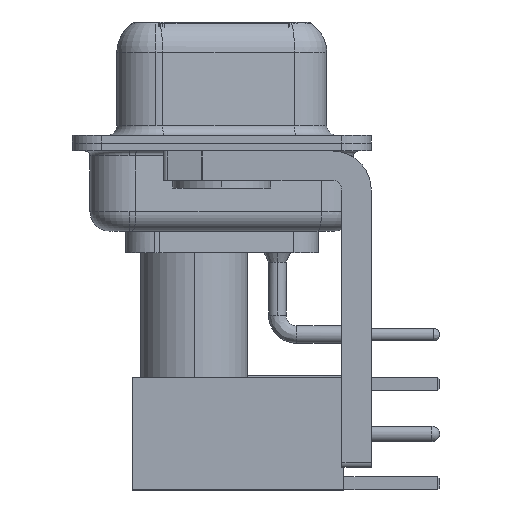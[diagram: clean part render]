
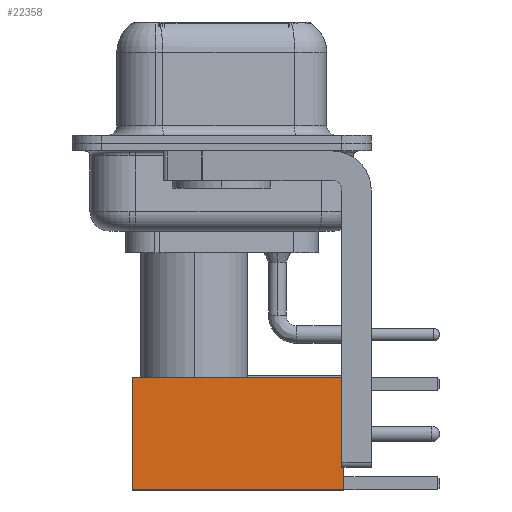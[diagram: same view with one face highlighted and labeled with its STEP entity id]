
A CAD part, left-side view. The second image highlights one B-rep face of the part: STEP entity #22358.
In plain terms, the highlighted face is planar.
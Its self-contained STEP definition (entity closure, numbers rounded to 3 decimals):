
#1876 = LINE ( 'NONE', #10668, #19207 ) ;
#3107 = CARTESIAN_POINT ( 'NONE',  ( 0., 2.875, 0. ) ) ;
#3415 = ORIENTED_EDGE ( 'NONE', *, *, #3549, .F. ) ;
#3437 = VERTEX_POINT ( 'NONE', #18532 ) ;
#3549 = EDGE_CURVE ( 'NONE', #3437, #8320, #31125, .T. ) ;
#3899 = DIRECTION ( 'NONE',  ( 0., 1., 0. ) ) ;
#5084 = EDGE_CURVE ( 'NONE', #8320, #7534, #14195, .T. ) ;
#5472 = DIRECTION ( 'NONE',  ( -1., 0., 0. ) ) ;
#5492 = DIRECTION ( 'NONE',  ( 0., 0., -1. ) ) ;
#7534 = VERTEX_POINT ( 'NONE', #22876 ) ;
#7855 = CARTESIAN_POINT ( 'NONE',  ( -2.875, 2.875, 0. ) ) ;
#8320 = VERTEX_POINT ( 'NONE', #27808 ) ;
#8653 = LINE ( 'NONE', #3107, #9652 ) ;
#9652 = VECTOR ( 'NONE', #37751, 1000. ) ;
#10668 = CARTESIAN_POINT ( 'NONE',  ( 2.875, 2.875, 0. ) ) ;
#12256 = AXIS2_PLACEMENT_3D ( 'NONE', #27830, #3899, #19214 ) ;
#14195 = LINE ( 'NONE', #7855, #32650 ) ;
#14318 = ORIENTED_EDGE ( 'NONE', *, *, #5084, .F. ) ;
#14774 = EDGE_CURVE ( 'NONE', #16494, #7534, #8653, .T. ) ;
#16494 = VERTEX_POINT ( 'NONE', #27989 ) ;
#17156 = VECTOR ( 'NONE', #5472, 1000. ) ;
#18532 = CARTESIAN_POINT ( 'NONE',  ( 2.875, 2.875, 10.82 ) ) ;
#18969 = EDGE_CURVE ( 'NONE', #3437, #16494, #1876, .T. ) ;
#19207 = VECTOR ( 'NONE', #5492, 1000. ) ;
#19214 = DIRECTION ( 'NONE',  ( 0., 0., 1. ) ) ;
#19590 = ORIENTED_EDGE ( 'NONE', *, *, #14774, .T. ) ;
#22358 = ADVANCED_FACE ( 'NONE', ( #23816 ), #35488, .T. ) ;
#22876 = CARTESIAN_POINT ( 'NONE',  ( -2.875, 2.875, 0. ) ) ;
#23816 = FACE_OUTER_BOUND ( 'NONE', #31026, .T. ) ;
#25391 = CARTESIAN_POINT ( 'NONE',  ( 0., 2.875, 10.82 ) ) ;
#25675 = DIRECTION ( 'NONE',  ( 0., 0., -1. ) ) ;
#27808 = CARTESIAN_POINT ( 'NONE',  ( -2.875, 2.875, 10.82 ) ) ;
#27830 = CARTESIAN_POINT ( 'NONE',  ( 2.875, 2.875, 0. ) ) ;
#27989 = CARTESIAN_POINT ( 'NONE',  ( 2.875, 2.875, 0. ) ) ;
#31026 = EDGE_LOOP ( 'NONE', ( #34446, #19590, #14318, #3415 ) ) ;
#31125 = LINE ( 'NONE', #25391, #17156 ) ;
#32650 = VECTOR ( 'NONE', #25675, 1000. ) ;
#34446 = ORIENTED_EDGE ( 'NONE', *, *, #18969, .T. ) ;
#35488 = PLANE ( 'NONE',  #12256 ) ;
#37751 = DIRECTION ( 'NONE',  ( -1., 0., 0. ) ) ;
